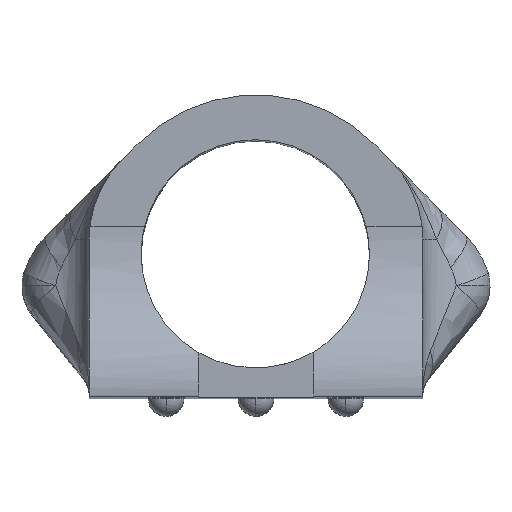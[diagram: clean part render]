
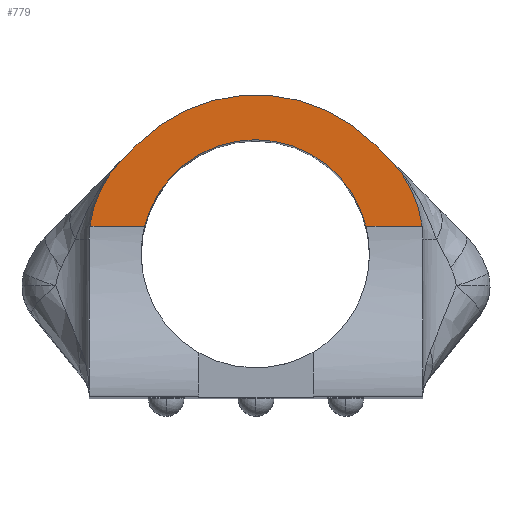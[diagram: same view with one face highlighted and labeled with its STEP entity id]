
A CAD part, top view. The second image highlights one B-rep face of the part: STEP entity #779.
In plain terms, the highlighted planar face has unit normal (0, 0, 1).
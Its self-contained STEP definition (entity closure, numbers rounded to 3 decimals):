
#18 = VERTEX_POINT ( 'NONE', #2264 ) ;
#282 = CARTESIAN_POINT ( 'NONE',  ( -1.632, 63.54, 46.922 ) ) ;
#328 = CARTESIAN_POINT ( 'NONE',  ( 10.687, 60.454, 46.922 ) ) ;
#333 = CIRCLE ( 'NONE', #755, 12.5 ) ;
#347 = CIRCLE ( 'NONE', #1903, 12.7 ) ;
#386 = AXIS2_PLACEMENT_3D ( 'NONE', #2491, #2256, #2251 ) ;
#486 = EDGE_CURVE ( 'NONE', #2125, #2658, #934, .T. ) ;
#572 = EDGE_CURVE ( 'NONE', #899, #2048, #920, .T. ) ;
#590 = ORIENTED_EDGE ( 'NONE', *, *, #2824, .T. ) ;
#667 = CARTESIAN_POINT ( 'NONE',  ( -4.142, 70.936, 46.922 ) ) ;
#684 = DIRECTION ( 'NONE',  ( 1., 0., 0. ) ) ;
#687 = DIRECTION ( 'NONE',  ( 0., 0., 1. ) ) ;
#694 = CARTESIAN_POINT ( 'NONE',  ( 4.697, 62.097, 46.922 ) ) ;
#705 = VECTOR ( 'NONE', #1059, 1000. ) ;
#714 = LINE ( 'NONE', #1079, #705 ) ;
#755 = AXIS2_PLACEMENT_3D ( 'NONE', #694, #687, #684 ) ;
#776 = DIRECTION ( 'NONE',  ( 0., 0., -1. ) ) ;
#779 = ADVANCED_FACE ( 'NONE', ( #842 ), #2289, .T. ) ;
#781 = CARTESIAN_POINT ( 'NONE',  ( 29.246, 63.54, 46.922 ) ) ;
#811 = CIRCLE ( 'NONE', #1332, 12.7 ) ;
#842 = FACE_OUTER_BOUND ( 'NONE', #1518, .T. ) ;
#899 = VERTEX_POINT ( 'NONE', #1975 ) ;
#920 = LINE ( 'NONE', #2687, #950 ) ;
#928 = VECTOR ( 'NONE', #2805, 1000. ) ;
#934 = LINE ( 'NONE', #2834, #928 ) ;
#939 = DIRECTION ( 'NONE',  ( 1., 0., 0. ) ) ;
#950 = VECTOR ( 'NONE', #2668, 1000. ) ;
#992 = DIRECTION ( 'NONE',  ( -1., 0., 0. ) ) ;
#1043 = EDGE_CURVE ( 'NONE', #1671, #1706, #714, .T. ) ;
#1051 = AXIS2_PLACEMENT_3D ( 'NONE', #3022, #2024, #1554 ) ;
#1059 = DIRECTION ( 'NONE',  ( -0.707, -0.707, 0. ) ) ;
#1079 = CARTESIAN_POINT ( 'NONE',  ( -2.371, 72.707, 46.922 ) ) ;
#1149 = ORIENTED_EDGE ( 'NONE', *, *, #572, .T. ) ;
#1155 = CARTESIAN_POINT ( 'NONE',  ( -2.371, 72.707, 46.922 ) ) ;
#1159 = CARTESIAN_POINT ( 'NONE',  ( 10.763, 59.573, 46.922 ) ) ;
#1166 = CARTESIAN_POINT ( 'NONE',  ( 23.006, 63.54, 46.922 ) ) ;
#1286 = CIRCLE ( 'NONE', #1541, 18.575 ) ;
#1330 = DIRECTION ( 'NONE',  ( 0., 0., -1. ) ) ;
#1332 = AXIS2_PLACEMENT_3D ( 'NONE', #328, #776, #1737 ) ;
#1353 = DIRECTION ( 'NONE',  ( 1., 0., 0. ) ) ;
#1371 = VECTOR ( 'NONE', #992, 1000. ) ;
#1518 = EDGE_LOOP ( 'NONE', ( #2908, #2057, #2792, #1758, #2912, #590, #1875, #2607, #1149 ) ) ;
#1541 = AXIS2_PLACEMENT_3D ( 'NONE', #1159, #2322, #1353 ) ;
#1554 = DIRECTION ( 'NONE',  ( 1., 0., 0. ) ) ;
#1577 = CARTESIAN_POINT ( 'NONE',  ( 10.687, 73.154, 46.922 ) ) ;
#1645 = EDGE_CURVE ( 'NONE', #1933, #2548, #347, .T. ) ;
#1671 = VERTEX_POINT ( 'NONE', #1155 ) ;
#1685 = EDGE_CURVE ( 'NONE', #1706, #18, #333, .T. ) ;
#1706 = VERTEX_POINT ( 'NONE', #667 ) ;
#1737 = DIRECTION ( 'NONE',  ( 1., 0., 0. ) ) ;
#1758 = ORIENTED_EDGE ( 'NONE', *, *, #2804, .F. ) ;
#1875 = ORIENTED_EDGE ( 'NONE', *, *, #486, .F. ) ;
#1903 = AXIS2_PLACEMENT_3D ( 'NONE', #3034, #1330, #939 ) ;
#1933 = VERTEX_POINT ( 'NONE', #282 ) ;
#1975 = CARTESIAN_POINT ( 'NONE',  ( 25.669, 70.936, 46.922 ) ) ;
#2024 = DIRECTION ( 'NONE',  ( 0., 0., 1. ) ) ;
#2048 = VERTEX_POINT ( 'NONE', #3001 ) ;
#2057 = ORIENTED_EDGE ( 'NONE', *, *, #1043, .T. ) ;
#2125 = VERTEX_POINT ( 'NONE', #781 ) ;
#2211 = CARTESIAN_POINT ( 'NONE',  ( 29.23, 63.54, 46.922 ) ) ;
#2230 = CIRCLE ( 'NONE', #1051, 12.5 ) ;
#2251 = DIRECTION ( 'NONE',  ( 1., 0., 0. ) ) ;
#2256 = DIRECTION ( 'NONE',  ( 0., 0., 1. ) ) ;
#2264 = CARTESIAN_POINT ( 'NONE',  ( -7.72, 63.54, 46.922 ) ) ;
#2289 = PLANE ( 'NONE',  #386 ) ;
#2322 = DIRECTION ( 'NONE',  ( 0., 0., 1. ) ) ;
#2419 = LINE ( 'NONE', #2211, #1371 ) ;
#2491 = CARTESIAN_POINT ( 'NONE',  ( 29.33, 38.127, 46.922 ) ) ;
#2548 = VERTEX_POINT ( 'NONE', #1577 ) ;
#2607 = ORIENTED_EDGE ( 'NONE', *, *, #3038, .T. ) ;
#2658 = VERTEX_POINT ( 'NONE', #1166 ) ;
#2668 = DIRECTION ( 'NONE',  ( -0.707, 0.707, 0. ) ) ;
#2669 = EDGE_CURVE ( 'NONE', #2048, #1671, #1286, .T. ) ;
#2687 = CARTESIAN_POINT ( 'NONE',  ( 29.33, 67.275, 46.922 ) ) ;
#2792 = ORIENTED_EDGE ( 'NONE', *, *, #1685, .T. ) ;
#2804 = EDGE_CURVE ( 'NONE', #1933, #18, #2419, .T. ) ;
#2805 = DIRECTION ( 'NONE',  ( -1., 0., 0. ) ) ;
#2824 = EDGE_CURVE ( 'NONE', #2548, #2658, #811, .T. ) ;
#2834 = CARTESIAN_POINT ( 'NONE',  ( 29.23, 63.54, 46.922 ) ) ;
#2908 = ORIENTED_EDGE ( 'NONE', *, *, #2669, .T. ) ;
#2912 = ORIENTED_EDGE ( 'NONE', *, *, #1645, .T. ) ;
#3001 = CARTESIAN_POINT ( 'NONE',  ( 23.898, 72.707, 46.922 ) ) ;
#3022 = CARTESIAN_POINT ( 'NONE',  ( 16.83, 62.097, 46.922 ) ) ;
#3034 = CARTESIAN_POINT ( 'NONE',  ( 10.687, 60.454, 46.922 ) ) ;
#3038 = EDGE_CURVE ( 'NONE', #2125, #899, #2230, .T. ) ;
